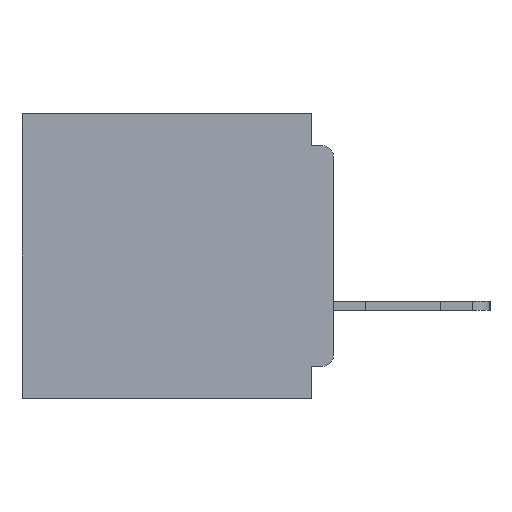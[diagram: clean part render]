
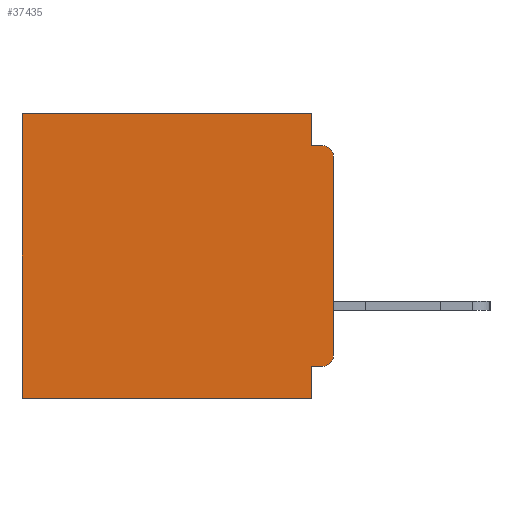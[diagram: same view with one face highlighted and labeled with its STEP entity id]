
A CAD part, left-side view. The second image highlights one B-rep face of the part: STEP entity #37435.
In plain terms, the highlighted planar face has unit normal (-1, 0, 0).
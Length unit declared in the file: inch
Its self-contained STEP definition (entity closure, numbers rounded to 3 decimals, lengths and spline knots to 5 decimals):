
#39 = VECTOR ( 'NONE', #5743, 39.37008 ) ;
#1076 = CARTESIAN_POINT ( 'NONE',  ( 0.3, 0.437, -0.4 ) ) ;
#1740 = AXIS2_PLACEMENT_3D ( 'NONE', #27789, #36220, #11150 ) ;
#1966 = ORIENTED_EDGE ( 'NONE', *, *, #9376, .T. ) ;
#2763 = ORIENTED_EDGE ( 'NONE', *, *, #7552, .F. ) ;
#3332 = EDGE_CURVE ( 'NONE', #17679, #13169, #18080, .T. ) ;
#3850 = VECTOR ( 'NONE', #37430, 39.37008 ) ;
#3871 = CARTESIAN_POINT ( 'NONE',  ( 0.3, 0., -0.355 ) ) ;
#5336 = DIRECTION ( 'NONE',  ( 0., 0., -1. ) ) ;
#5743 = DIRECTION ( 'NONE',  ( 0., 1., 0. ) ) ;
#5955 = VERTEX_POINT ( 'NONE', #46723 ) ;
#6783 = VERTEX_POINT ( 'NONE', #34263 ) ;
#6902 = PLANE ( 'NONE',  #1740 ) ;
#7552 = EDGE_CURVE ( 'NONE', #30947, #23009, #43887, .T. ) ;
#9376 = EDGE_CURVE ( 'NONE', #5955, #48722, #28557, .T. ) ;
#9405 = EDGE_CURVE ( 'NONE', #23009, #11619, #46943, .T. ) ;
#9629 = ORIENTED_EDGE ( 'NONE', *, *, #51547, .T. ) ;
#11150 = DIRECTION ( 'NONE',  ( 0., 0., -1. ) ) ;
#11619 = VERTEX_POINT ( 'NONE', #27427 ) ;
#11724 = CARTESIAN_POINT ( 'NONE',  ( 0.3, 0., -0.06 ) ) ;
#11965 = AXIS2_PLACEMENT_3D ( 'NONE', #19016, #48402, #23243 ) ;
#12028 = ORIENTED_EDGE ( 'NONE', *, *, #12089, .T. ) ;
#12089 = EDGE_CURVE ( 'NONE', #17679, #6783, #21075, .T. ) ;
#13169 = VERTEX_POINT ( 'NONE', #25794 ) ;
#13541 = ORIENTED_EDGE ( 'NONE', *, *, #47307, .F. ) ;
#14760 = VECTOR ( 'NONE', #19197, 39.37008 ) ;
#15281 = CARTESIAN_POINT ( 'NONE',  ( 0.3, 0., -0.34 ) ) ;
#15655 = DIRECTION ( 'NONE',  ( 0., 0., -1. ) ) ;
#16756 = ORIENTED_EDGE ( 'NONE', *, *, #9405, .F. ) ;
#17679 = VERTEX_POINT ( 'NONE', #33057 ) ;
#18080 = LINE ( 'NONE', #38690, #50258 ) ;
#19016 = CARTESIAN_POINT ( 'NONE',  ( 0.3, 0.015, -0.34 ) ) ;
#19196 = VECTOR ( 'NONE', #15655, 39.37008 ) ;
#19197 = DIRECTION ( 'NONE',  ( 0., 1., 0. ) ) ;
#20962 = CARTESIAN_POINT ( 'NONE',  ( 0.3, 0.015, -0.06 ) ) ;
#21075 = LINE ( 'NONE', #39315, #39 ) ;
#21091 = EDGE_CURVE ( 'NONE', #5955, #30947, #24835, .T. ) ;
#21605 = VERTEX_POINT ( 'NONE', #11724 ) ;
#21851 = FACE_OUTER_BOUND ( 'NONE', #44450, .T. ) ;
#23009 = VERTEX_POINT ( 'NONE', #29151 ) ;
#23116 = LINE ( 'NONE', #1076, #34272 ) ;
#23243 = DIRECTION ( 'NONE',  ( 0., 0., -1. ) ) ;
#24585 = AXIS2_PLACEMENT_3D ( 'NONE', #20962, #50325, #25196 ) ;
#24835 = LINE ( 'NONE', #3871, #3850 ) ;
#25196 = DIRECTION ( 'NONE',  ( 0., 0., -1. ) ) ;
#25575 = VECTOR ( 'NONE', #41058, 39.37008 ) ;
#25794 = CARTESIAN_POINT ( 'NONE',  ( 0.3, 0.031, -0.045 ) ) ;
#26002 = VERTEX_POINT ( 'NONE', #47520 ) ;
#26901 = LINE ( 'NONE', #45275, #25575 ) ;
#27015 = EDGE_CURVE ( 'NONE', #21605, #26002, #44905, .T. ) ;
#27427 = CARTESIAN_POINT ( 'NONE',  ( 0.3, 0.437, -0.4 ) ) ;
#27789 = CARTESIAN_POINT ( 'NONE',  ( 0.3, 0., -0.4 ) ) ;
#28557 = CIRCLE ( 'NONE', #11965, 0.015 ) ;
#29151 = CARTESIAN_POINT ( 'NONE',  ( 0.3, 0.031, -0.4 ) ) ;
#30947 = VERTEX_POINT ( 'NONE', #50985 ) ;
#31419 = VECTOR ( 'NONE', #32586, 39.37008 ) ;
#32586 = DIRECTION ( 'NONE',  ( 0., 0., -1. ) ) ;
#33057 = CARTESIAN_POINT ( 'NONE',  ( 0.3, 0.031, 0. ) ) ;
#33185 = CARTESIAN_POINT ( 'NONE',  ( 0.3, 0.031, -0.4 ) ) ;
#33923 = ORIENTED_EDGE ( 'NONE', *, *, #27015, .T. ) ;
#34263 = CARTESIAN_POINT ( 'NONE',  ( 0.3, 0.437, 0. ) ) ;
#34272 = VECTOR ( 'NONE', #5336, 39.37008 ) ;
#36220 = DIRECTION ( 'NONE',  ( 1., 0., 0. ) ) ;
#37369 = ORIENTED_EDGE ( 'NONE', *, *, #21091, .F. ) ;
#37430 = DIRECTION ( 'NONE',  ( 0., 1., 0. ) ) ;
#37435 = ADVANCED_FACE ( 'NONE', ( #21851 ), #6902, .F. ) ;
#37490 = EDGE_CURVE ( 'NONE', #21605, #48722, #38926, .T. ) ;
#38690 = CARTESIAN_POINT ( 'NONE',  ( 0.3, 0.031, 0. ) ) ;
#38926 = LINE ( 'NONE', #40828, #19196 ) ;
#39042 = ORIENTED_EDGE ( 'NONE', *, *, #3332, .F. ) ;
#39315 = CARTESIAN_POINT ( 'NONE',  ( 0.3, 0., 0. ) ) ;
#39836 = ORIENTED_EDGE ( 'NONE', *, *, #37490, .F. ) ;
#40828 = CARTESIAN_POINT ( 'NONE',  ( 0.3, 0., -0.4 ) ) ;
#41058 = DIRECTION ( 'NONE',  ( 0., -1., 0. ) ) ;
#43887 = LINE ( 'NONE', #33185, #31419 ) ;
#44450 = EDGE_LOOP ( 'NONE', ( #39836, #33923, #13541, #39042, #12028, #9629, #16756, #2763, #37369, #1966 ) ) ;
#44905 = CIRCLE ( 'NONE', #24585, 0.015 ) ;
#45275 = CARTESIAN_POINT ( 'NONE',  ( 0.3, 0., -0.045 ) ) ;
#46723 = CARTESIAN_POINT ( 'NONE',  ( 0.3, 0.015, -0.355 ) ) ;
#46943 = LINE ( 'NONE', #48578, #14760 ) ;
#47307 = EDGE_CURVE ( 'NONE', #13169, #26002, #26901, .T. ) ;
#47520 = CARTESIAN_POINT ( 'NONE',  ( 0.3, 0.015, -0.045 ) ) ;
#48402 = DIRECTION ( 'NONE',  ( -1., 0., 0. ) ) ;
#48578 = CARTESIAN_POINT ( 'NONE',  ( 0.3, 0., -0.4 ) ) ;
#48722 = VERTEX_POINT ( 'NONE', #15281 ) ;
#50258 = VECTOR ( 'NONE', #52839, 39.37008 ) ;
#50325 = DIRECTION ( 'NONE',  ( -1., 0., 0. ) ) ;
#50985 = CARTESIAN_POINT ( 'NONE',  ( 0.3, 0.031, -0.355 ) ) ;
#51547 = EDGE_CURVE ( 'NONE', #6783, #11619, #23116, .T. ) ;
#52839 = DIRECTION ( 'NONE',  ( 0., 0., -1. ) ) ;
